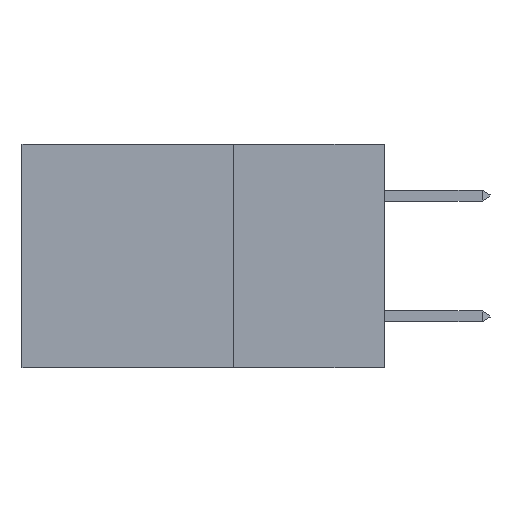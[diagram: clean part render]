
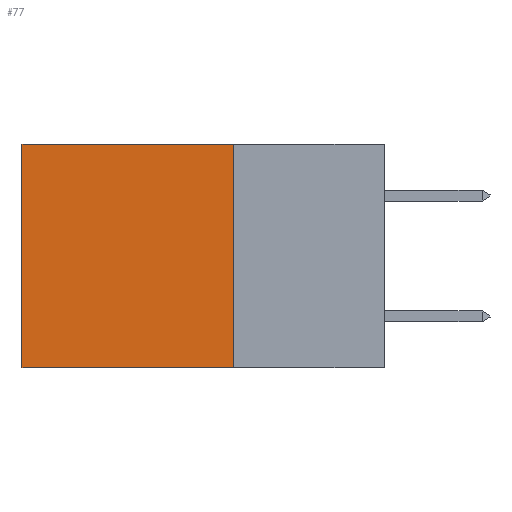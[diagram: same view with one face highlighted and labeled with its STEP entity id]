
A CAD part, left-side view. The second image highlights one B-rep face of the part: STEP entity #77.
In plain terms, the highlighted planar face has unit normal (-1, 0, 0).
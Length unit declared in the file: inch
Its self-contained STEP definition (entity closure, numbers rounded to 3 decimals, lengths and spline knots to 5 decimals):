
#77 = ADVANCED_FACE ( 'NONE', ( #11200 ), #8999, .F. ) ;
#513 = CARTESIAN_POINT ( 'NONE',  ( 0.2875, 0.25, 0. ) ) ;
#810 = VERTEX_POINT ( 'NONE', #4098 ) ;
#1482 = CARTESIAN_POINT ( 'NONE',  ( 0.2875, 0.6, 0. ) ) ;
#3252 = EDGE_CURVE ( 'NONE', #4534, #810, #15681, .T. ) ;
#4098 = CARTESIAN_POINT ( 'NONE',  ( 0.2875, 0.6, -0.37 ) ) ;
#4193 = CARTESIAN_POINT ( 'NONE',  ( 0.2875, 0.25, -0.37 ) ) ;
#4240 = EDGE_CURVE ( 'NONE', #12300, #4534, #11073, .T. ) ;
#4534 = VERTEX_POINT ( 'NONE', #10529 ) ;
#4925 = CARTESIAN_POINT ( 'NONE',  ( 0.2875, 0.25, 0. ) ) ;
#5127 = EDGE_CURVE ( 'NONE', #12300, #15937, #18382, .T. ) ;
#5595 = EDGE_CURVE ( 'NONE', #15937, #810, #11023, .T. ) ;
#8744 = CARTESIAN_POINT ( 'NONE',  ( 0.2875, 0.25, -0.37 ) ) ;
#8999 = PLANE ( 'NONE',  #13968 ) ;
#9187 = DIRECTION ( 'NONE',  ( 0., 0., -1. ) ) ;
#10529 = CARTESIAN_POINT ( 'NONE',  ( 0.2875, 0.6, 0. ) ) ;
#10888 = ORIENTED_EDGE ( 'NONE', *, *, #5595, .F. ) ;
#11023 = LINE ( 'NONE', #4193, #15907 ) ;
#11073 = LINE ( 'NONE', #17542, #22982 ) ;
#11200 = FACE_OUTER_BOUND ( 'NONE', #20909, .T. ) ;
#12300 = VERTEX_POINT ( 'NONE', #4925 ) ;
#13579 = ORIENTED_EDGE ( 'NONE', *, *, #5127, .F. ) ;
#13968 = AXIS2_PLACEMENT_3D ( 'NONE', #14763, #14934, #9187 ) ;
#14763 = CARTESIAN_POINT ( 'NONE',  ( 0.2875, 0.25, 0. ) ) ;
#14934 = DIRECTION ( 'NONE',  ( 1., 0., 0. ) ) ;
#15107 = DIRECTION ( 'NONE',  ( 0., 0., -1. ) ) ;
#15681 = LINE ( 'NONE', #1482, #24855 ) ;
#15907 = VECTOR ( 'NONE', #15926, 39.37008 ) ;
#15926 = DIRECTION ( 'NONE',  ( 0., 1., 0. ) ) ;
#15937 = VERTEX_POINT ( 'NONE', #8744 ) ;
#16842 = VECTOR ( 'NONE', #18352, 39.37008 ) ;
#17542 = CARTESIAN_POINT ( 'NONE',  ( 0.2875, 0.25, 0. ) ) ;
#18352 = DIRECTION ( 'NONE',  ( 0., 0., -1. ) ) ;
#18382 = LINE ( 'NONE', #513, #16842 ) ;
#19207 = DIRECTION ( 'NONE',  ( 0., 1., 0. ) ) ;
#20301 = ORIENTED_EDGE ( 'NONE', *, *, #4240, .T. ) ;
#20909 = EDGE_LOOP ( 'NONE', ( #22843, #10888, #13579, #20301 ) ) ;
#22843 = ORIENTED_EDGE ( 'NONE', *, *, #3252, .T. ) ;
#22982 = VECTOR ( 'NONE', #19207, 39.37008 ) ;
#24855 = VECTOR ( 'NONE', #15107, 39.37008 ) ;
